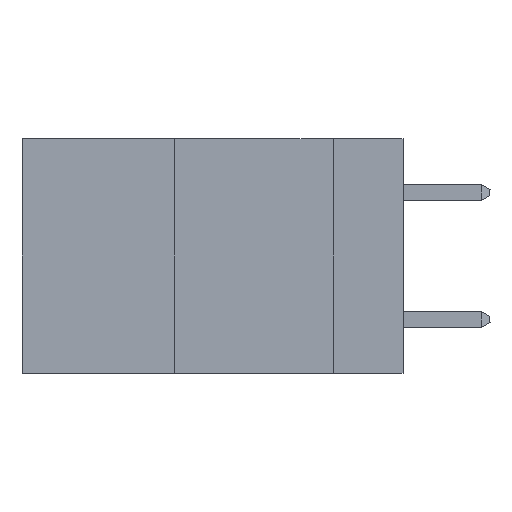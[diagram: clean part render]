
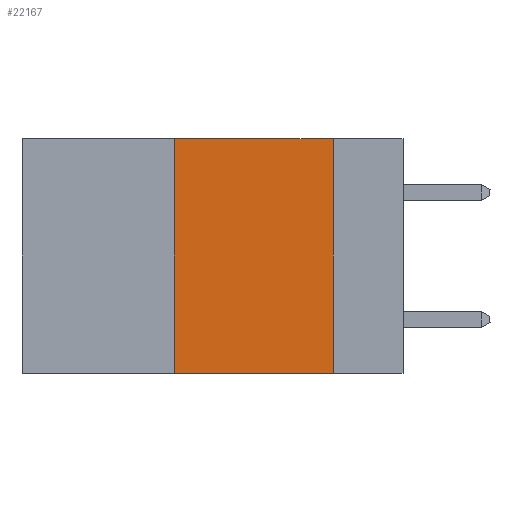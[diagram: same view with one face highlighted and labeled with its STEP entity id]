
A CAD part, left-side view. The second image highlights one B-rep face of the part: STEP entity #22167.
In plain terms, the highlighted planar face has unit normal (-1, 0, 0).
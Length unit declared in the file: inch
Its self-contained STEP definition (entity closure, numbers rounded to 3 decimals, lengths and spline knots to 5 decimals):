
#2084 = ORIENTED_EDGE ( 'NONE', *, *, #15230, .F. ) ;
#2737 = VERTEX_POINT ( 'NONE', #5500 ) ;
#3171 = VECTOR ( 'NONE', #13522, 39.37008 ) ;
#3828 = LINE ( 'NONE', #11451, #3171 ) ;
#4516 = EDGE_LOOP ( 'NONE', ( #2084, #7602, #13053, #19799 ) ) ;
#4577 = VERTEX_POINT ( 'NONE', #17600 ) ;
#4705 = VECTOR ( 'NONE', #13025, 39.37008 ) ;
#5500 = CARTESIAN_POINT ( 'NONE',  ( 0., 0.11, -0.37 ) ) ;
#6100 = PLANE ( 'NONE',  #21709 ) ;
#7602 = ORIENTED_EDGE ( 'NONE', *, *, #13758, .F. ) ;
#8917 = DIRECTION ( 'NONE',  ( 0., 0., 1. ) ) ;
#10241 = CARTESIAN_POINT ( 'NONE',  ( 0., 0.6, 0. ) ) ;
#10747 = LINE ( 'NONE', #13623, #21047 ) ;
#11451 = CARTESIAN_POINT ( 'NONE',  ( 0., 0.6, 0. ) ) ;
#12163 = LINE ( 'NONE', #19146, #22424 ) ;
#12294 = DIRECTION ( 'NONE',  ( 0., 0., -1. ) ) ;
#13025 = DIRECTION ( 'NONE',  ( 0., 0., -1. ) ) ;
#13053 = ORIENTED_EDGE ( 'NONE', *, *, #14291, .F. ) ;
#13180 = FACE_OUTER_BOUND ( 'NONE', #4516, .T. ) ;
#13522 = DIRECTION ( 'NONE',  ( 0., -1., 0. ) ) ;
#13623 = CARTESIAN_POINT ( 'NONE',  ( 0., 0.6, -0.37 ) ) ;
#13758 = EDGE_CURVE ( 'NONE', #22306, #15205, #3828, .T. ) ;
#14291 = EDGE_CURVE ( 'NONE', #4577, #22306, #12163, .T. ) ;
#14969 = CARTESIAN_POINT ( 'NONE',  ( 0., 0.36, 0. ) ) ;
#15205 = VERTEX_POINT ( 'NONE', #19031 ) ;
#15230 = EDGE_CURVE ( 'NONE', #15205, #2737, #16259, .T. ) ;
#15669 = DIRECTION ( 'NONE',  ( 0., -1., 0. ) ) ;
#16095 = EDGE_CURVE ( 'NONE', #4577, #2737, #10747, .T. ) ;
#16259 = LINE ( 'NONE', #23212, #4705 ) ;
#17600 = CARTESIAN_POINT ( 'NONE',  ( 0., 0.36, -0.37 ) ) ;
#19031 = CARTESIAN_POINT ( 'NONE',  ( 0., 0.11, 0. ) ) ;
#19146 = CARTESIAN_POINT ( 'NONE',  ( 0., 0.36, 0. ) ) ;
#19799 = ORIENTED_EDGE ( 'NONE', *, *, #16095, .T. ) ;
#21047 = VECTOR ( 'NONE', #15669, 39.37008 ) ;
#21709 = AXIS2_PLACEMENT_3D ( 'NONE', #10241, #24502, #12294 ) ;
#22167 = ADVANCED_FACE ( 'NONE', ( #13180 ), #6100, .F. ) ;
#22306 = VERTEX_POINT ( 'NONE', #14969 ) ;
#22424 = VECTOR ( 'NONE', #8917, 39.37008 ) ;
#23212 = CARTESIAN_POINT ( 'NONE',  ( 0., 0.11, 0. ) ) ;
#24502 = DIRECTION ( 'NONE',  ( 1., 0., 0. ) ) ;
